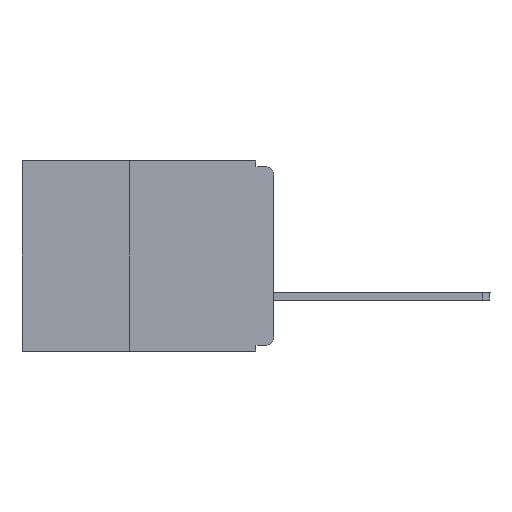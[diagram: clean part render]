
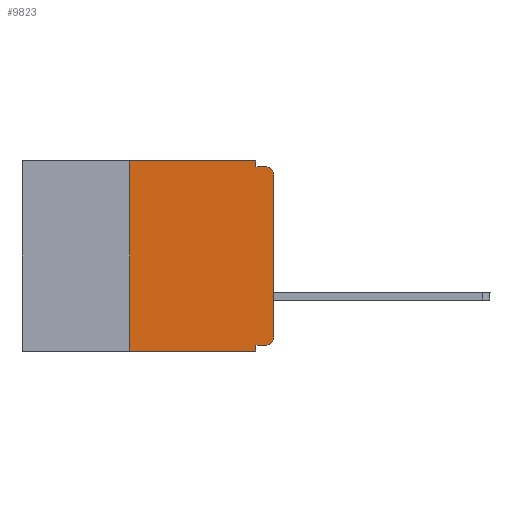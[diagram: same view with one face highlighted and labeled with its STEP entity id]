
A CAD part, left-side view. The second image highlights one B-rep face of the part: STEP entity #9823.
In plain terms, the highlighted planar face has unit normal (-1, 0, 0).
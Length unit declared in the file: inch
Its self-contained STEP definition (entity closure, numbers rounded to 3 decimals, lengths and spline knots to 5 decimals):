
#16 = AXIS2_PLACEMENT_3D ( 'NONE', #6339, #120, #3953 ) ;
#120 = DIRECTION ( 'NONE',  ( -1., 0., 0. ) ) ;
#308 = CARTESIAN_POINT ( 'NONE',  ( 0., 0.25, -0.33 ) ) ;
#600 = EDGE_LOOP ( 'NONE', ( #6681, #10998, #5994, #5488, #13251, #3086, #4230, #2293, #7226, #911 ) ) ;
#707 = VERTEX_POINT ( 'NONE', #8066 ) ;
#895 = EDGE_CURVE ( 'NONE', #12061, #7994, #6986, .T. ) ;
#911 = ORIENTED_EDGE ( 'NONE', *, *, #2857, .T. ) ;
#1413 = CARTESIAN_POINT ( 'NONE',  ( 0., 0.015, -0.01 ) ) ;
#1818 = LINE ( 'NONE', #9548, #8862 ) ;
#1821 = AXIS2_PLACEMENT_3D ( 'NONE', #14560, #12141, #5843 ) ;
#2029 = VECTOR ( 'NONE', #12674, 39.37008 ) ;
#2293 = ORIENTED_EDGE ( 'NONE', *, *, #7733, .F. ) ;
#2379 = LINE ( 'NONE', #2512, #14069 ) ;
#2512 = CARTESIAN_POINT ( 'NONE',  ( 0., 0.031, -0.33 ) ) ;
#2674 = CARTESIAN_POINT ( 'NONE',  ( 0., 0., -0.305 ) ) ;
#2857 = EDGE_CURVE ( 'NONE', #13507, #12534, #6201, .T. ) ;
#2928 = CARTESIAN_POINT ( 'NONE',  ( 0., 0., -0.32 ) ) ;
#3019 = CARTESIAN_POINT ( 'NONE',  ( 0., 0.015, -0.32 ) ) ;
#3039 = VECTOR ( 'NONE', #13850, 39.37008 ) ;
#3086 = ORIENTED_EDGE ( 'NONE', *, *, #13409, .F. ) ;
#3698 = DIRECTION ( 'NONE',  ( 0., 0., -1. ) ) ;
#3701 = VECTOR ( 'NONE', #11079, 39.37008 ) ;
#3795 = VERTEX_POINT ( 'NONE', #1413 ) ;
#3953 = DIRECTION ( 'NONE',  ( 0., 0., -1. ) ) ;
#4182 = VECTOR ( 'NONE', #11253, 39.37008 ) ;
#4230 = ORIENTED_EDGE ( 'NONE', *, *, #895, .T. ) ;
#4397 = EDGE_CURVE ( 'NONE', #14058, #707, #5743, .T. ) ;
#4488 = CARTESIAN_POINT ( 'NONE',  ( 0., 0., -0.025 ) ) ;
#4781 = LINE ( 'NONE', #15772, #12025 ) ;
#4912 = PLANE ( 'NONE',  #15732 ) ;
#4967 = CARTESIAN_POINT ( 'NONE',  ( 0., 0.437, 0. ) ) ;
#5488 = ORIENTED_EDGE ( 'NONE', *, *, #13481, .F. ) ;
#5743 = LINE ( 'NONE', #4967, #4182 ) ;
#5753 = CARTESIAN_POINT ( 'NONE',  ( 0., 0.031, -0.32 ) ) ;
#5843 = DIRECTION ( 'NONE',  ( 0., 0., -1. ) ) ;
#5933 = EDGE_CURVE ( 'NONE', #8191, #3795, #8645, .T. ) ;
#5994 = ORIENTED_EDGE ( 'NONE', *, *, #14705, .F. ) ;
#6201 = CIRCLE ( 'NONE', #16, 0.015 ) ;
#6339 = CARTESIAN_POINT ( 'NONE',  ( 0., 0.015, -0.305 ) ) ;
#6681 = ORIENTED_EDGE ( 'NONE', *, *, #15760, .T. ) ;
#6986 = LINE ( 'NONE', #11187, #3701 ) ;
#7226 = ORIENTED_EDGE ( 'NONE', *, *, #9509, .F. ) ;
#7322 = CARTESIAN_POINT ( 'NONE',  ( 0., 0.031, -0.01 ) ) ;
#7422 = DIRECTION ( 'NONE',  ( 0., 0., -1. ) ) ;
#7439 = VECTOR ( 'NONE', #13004, 39.37008 ) ;
#7472 = LINE ( 'NONE', #8807, #2029 ) ;
#7733 = EDGE_CURVE ( 'NONE', #14033, #7994, #2379, .T. ) ;
#7994 = VERTEX_POINT ( 'NONE', #8528 ) ;
#8066 = CARTESIAN_POINT ( 'NONE',  ( 0., 0.031, 0. ) ) ;
#8191 = VERTEX_POINT ( 'NONE', #4488 ) ;
#8398 = CARTESIAN_POINT ( 'NONE',  ( 0., 0.25, 0. ) ) ;
#8528 = CARTESIAN_POINT ( 'NONE',  ( 0., 0.031, -0.33 ) ) ;
#8645 = CIRCLE ( 'NONE', #1821, 0.015 ) ;
#8807 = CARTESIAN_POINT ( 'NONE',  ( 0., 0., -0.01 ) ) ;
#8862 = VECTOR ( 'NONE', #10973, 39.37008 ) ;
#9509 = EDGE_CURVE ( 'NONE', #13507, #14033, #13535, .T. ) ;
#9548 = CARTESIAN_POINT ( 'NONE',  ( 0., 0., 0. ) ) ;
#9806 = DIRECTION ( 'NONE',  ( 0., 0., -1. ) ) ;
#9823 = ADVANCED_FACE ( 'NONE', ( #14295 ), #4912, .F. ) ;
#10904 = CARTESIAN_POINT ( 'NONE',  ( 0., 0.25, -0.33 ) ) ;
#10973 = DIRECTION ( 'NONE',  ( 0., 0., 1. ) ) ;
#10998 = ORIENTED_EDGE ( 'NONE', *, *, #5933, .T. ) ;
#11079 = DIRECTION ( 'NONE',  ( 0., -1., 0. ) ) ;
#11184 = VERTEX_POINT ( 'NONE', #7322 ) ;
#11187 = CARTESIAN_POINT ( 'NONE',  ( 0., 0.437, -0.33 ) ) ;
#11253 = DIRECTION ( 'NONE',  ( 0., -1., 0. ) ) ;
#12025 = VECTOR ( 'NONE', #9806, 39.37008 ) ;
#12061 = VERTEX_POINT ( 'NONE', #10904 ) ;
#12141 = DIRECTION ( 'NONE',  ( -1., 0., 0. ) ) ;
#12534 = VERTEX_POINT ( 'NONE', #2674 ) ;
#12674 = DIRECTION ( 'NONE',  ( 0., -1., 0. ) ) ;
#13004 = DIRECTION ( 'NONE',  ( 0., 1., 0. ) ) ;
#13251 = ORIENTED_EDGE ( 'NONE', *, *, #4397, .F. ) ;
#13409 = EDGE_CURVE ( 'NONE', #12061, #14058, #15358, .T. ) ;
#13481 = EDGE_CURVE ( 'NONE', #707, #11184, #4781, .T. ) ;
#13507 = VERTEX_POINT ( 'NONE', #3019 ) ;
#13535 = LINE ( 'NONE', #2928, #7439 ) ;
#13673 = CARTESIAN_POINT ( 'NONE',  ( 0., 0.437, 0. ) ) ;
#13850 = DIRECTION ( 'NONE',  ( 0., 0., 1. ) ) ;
#14033 = VERTEX_POINT ( 'NONE', #5753 ) ;
#14058 = VERTEX_POINT ( 'NONE', #8398 ) ;
#14069 = VECTOR ( 'NONE', #3698, 39.37008 ) ;
#14295 = FACE_OUTER_BOUND ( 'NONE', #600, .T. ) ;
#14560 = CARTESIAN_POINT ( 'NONE',  ( 0., 0.015, -0.025 ) ) ;
#14705 = EDGE_CURVE ( 'NONE', #11184, #3795, #7472, .T. ) ;
#14944 = DIRECTION ( 'NONE',  ( 1., 0., 0. ) ) ;
#15358 = LINE ( 'NONE', #308, #3039 ) ;
#15732 = AXIS2_PLACEMENT_3D ( 'NONE', #13673, #14944, #7422 ) ;
#15760 = EDGE_CURVE ( 'NONE', #12534, #8191, #1818, .T. ) ;
#15772 = CARTESIAN_POINT ( 'NONE',  ( 0., 0.031, 0. ) ) ;
